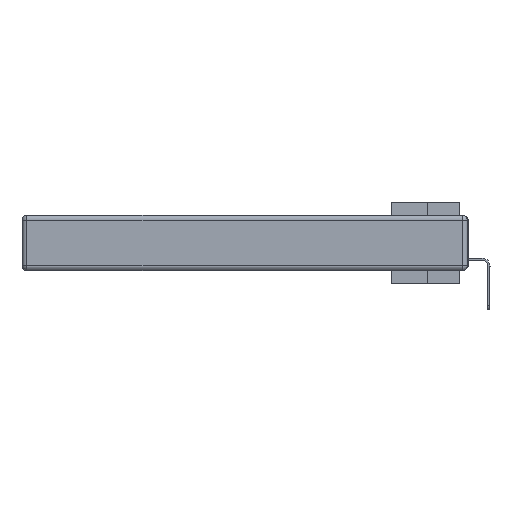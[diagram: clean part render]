
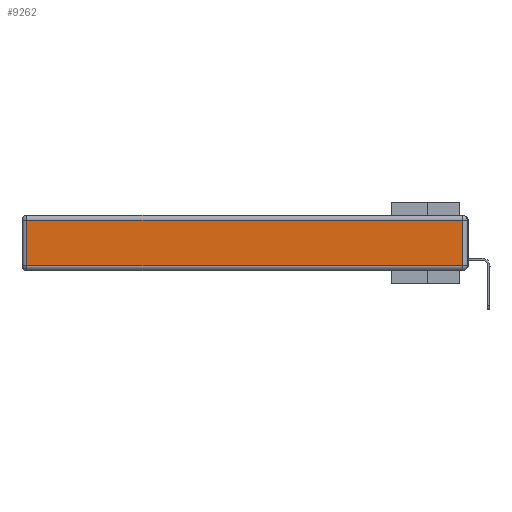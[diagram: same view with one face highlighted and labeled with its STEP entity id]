
A CAD part, left-side view. The second image highlights one B-rep face of the part: STEP entity #9262.
In plain terms, the highlighted planar face has unit normal (-1, 0, 0).
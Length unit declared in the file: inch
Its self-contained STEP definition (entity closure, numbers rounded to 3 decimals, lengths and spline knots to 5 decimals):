
#474 = DIRECTION ( 'NONE',  ( 0., 0., -1. ) ) ;
#855 = EDGE_CURVE ( 'NONE', #27474, #12507, #21620, .T. ) ;
#976 = DIRECTION ( 'NONE',  ( 0., 0., 1. ) ) ;
#2997 = EDGE_CURVE ( 'NONE', #12507, #21757, #21142, .T. ) ;
#3199 = LINE ( 'NONE', #22599, #21871 ) ;
#3679 = EDGE_CURVE ( 'NONE', #20359, #27474, #3199, .T. ) ;
#3794 = CARTESIAN_POINT ( 'NONE',  ( 0., 2.72, -0.313 ) ) ;
#4475 = VECTOR ( 'NONE', #22296, 39.37008 ) ;
#4612 = PLANE ( 'NONE',  #21364 ) ;
#5809 = ORIENTED_EDGE ( 'NONE', *, *, #2997, .T. ) ;
#6852 = EDGE_CURVE ( 'NONE', #21757, #20359, #23879, .T. ) ;
#9262 = ADVANCED_FACE ( 'NONE', ( #18362 ), #4612, .T. ) ;
#10823 = DIRECTION ( 'NONE',  ( -1., 0., 0. ) ) ;
#12507 = VERTEX_POINT ( 'NONE', #16002 ) ;
#12702 = ORIENTED_EDGE ( 'NONE', *, *, #6852, .T. ) ;
#14734 = CARTESIAN_POINT ( 'NONE',  ( 0., 0., -0.313 ) ) ;
#15063 = VECTOR ( 'NONE', #976, 39.37008 ) ;
#15186 = DIRECTION ( 'NONE',  ( 0., 0., 1. ) ) ;
#15541 = CARTESIAN_POINT ( 'NONE',  ( 0., 0.03, -0.343 ) ) ;
#15978 = ORIENTED_EDGE ( 'NONE', *, *, #855, .T. ) ;
#16002 = CARTESIAN_POINT ( 'NONE',  ( 0., 0.03, -0.313 ) ) ;
#17402 = VECTOR ( 'NONE', #20105, 39.37008 ) ;
#18362 = FACE_OUTER_BOUND ( 'NONE', #21776, .T. ) ;
#20105 = DIRECTION ( 'NONE',  ( 0., 1., 0. ) ) ;
#20305 = CARTESIAN_POINT ( 'NONE',  ( 0., 2.75, -0.03 ) ) ;
#20359 = VERTEX_POINT ( 'NONE', #22435 ) ;
#21142 = LINE ( 'NONE', #15541, #15063 ) ;
#21364 = AXIS2_PLACEMENT_3D ( 'NONE', #24881, #10823, #15186 ) ;
#21598 = CARTESIAN_POINT ( 'NONE',  ( 0., 0.03, -0.03 ) ) ;
#21620 = LINE ( 'NONE', #14734, #4475 ) ;
#21757 = VERTEX_POINT ( 'NONE', #21598 ) ;
#21776 = EDGE_LOOP ( 'NONE', ( #15978, #5809, #12702, #23746 ) ) ;
#21871 = VECTOR ( 'NONE', #474, 39.37008 ) ;
#22296 = DIRECTION ( 'NONE',  ( 0., -1., 0. ) ) ;
#22435 = CARTESIAN_POINT ( 'NONE',  ( 0., 2.72, -0.03 ) ) ;
#22599 = CARTESIAN_POINT ( 'NONE',  ( 0., 2.72, -0.343 ) ) ;
#23746 = ORIENTED_EDGE ( 'NONE', *, *, #3679, .T. ) ;
#23879 = LINE ( 'NONE', #20305, #17402 ) ;
#24881 = CARTESIAN_POINT ( 'NONE',  ( 0., 0., -0.343 ) ) ;
#27474 = VERTEX_POINT ( 'NONE', #3794 ) ;
